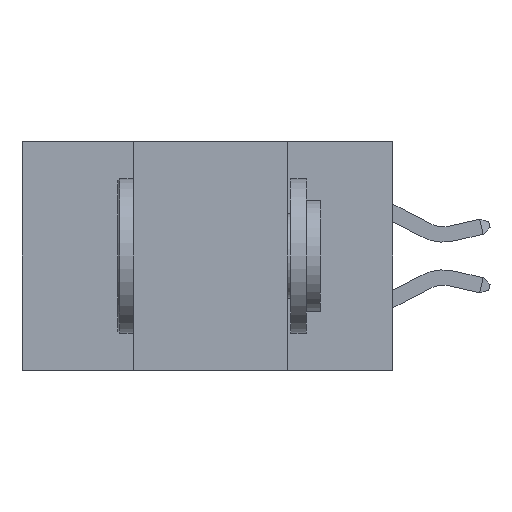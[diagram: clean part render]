
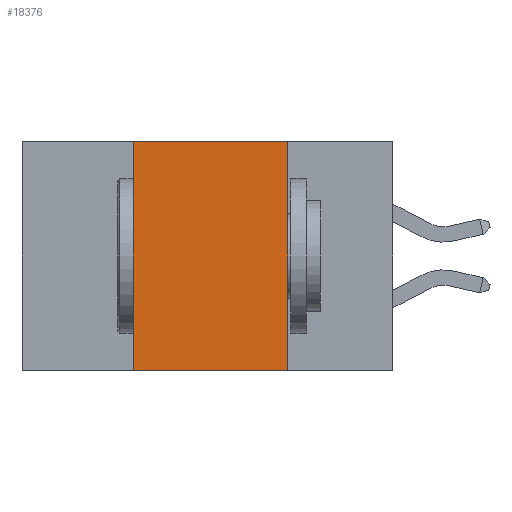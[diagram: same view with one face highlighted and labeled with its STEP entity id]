
A CAD part, left-side view. The second image highlights one B-rep face of the part: STEP entity #18376.
In plain terms, the highlighted planar face has unit normal (-1, 0, 0).
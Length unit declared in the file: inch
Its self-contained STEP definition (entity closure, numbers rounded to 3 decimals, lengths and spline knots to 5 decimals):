
#164 = ORIENTED_EDGE ( 'NONE', *, *, #11476, .F. ) ;
#1396 = EDGE_LOOP ( 'NONE', ( #15743, #164, #21096, #26042 ) ) ;
#4524 = VECTOR ( 'NONE', #17876, 39.37008 ) ;
#4577 = DIRECTION ( 'NONE',  ( 1., 0., 0. ) ) ;
#4940 = LINE ( 'NONE', #6911, #35645 ) ;
#5086 = CARTESIAN_POINT ( 'NONE',  ( 0., 0.6, -0.37 ) ) ;
#5673 = LINE ( 'NONE', #18594, #25231 ) ;
#6781 = DIRECTION ( 'NONE',  ( 0., -1., 0. ) ) ;
#6911 = CARTESIAN_POINT ( 'NONE',  ( 0., 0.6, 0. ) ) ;
#7108 = EDGE_CURVE ( 'NONE', #28613, #36774, #5673, .T. ) ;
#7483 = CARTESIAN_POINT ( 'NONE',  ( 0., 0.6, 0. ) ) ;
#7971 = EDGE_CURVE ( 'NONE', #33020, #36774, #28387, .T. ) ;
#11476 = EDGE_CURVE ( 'NONE', #26983, #28613, #4940, .T. ) ;
#12858 = FACE_OUTER_BOUND ( 'NONE', #1396, .T. ) ;
#13036 = DIRECTION ( 'NONE',  ( 0., 0., -1. ) ) ;
#14779 = CARTESIAN_POINT ( 'NONE',  ( 0., 0.17, -0.37 ) ) ;
#15743 = ORIENTED_EDGE ( 'NONE', *, *, #7108, .F. ) ;
#17222 = VECTOR ( 'NONE', #35237, 39.37008 ) ;
#17876 = DIRECTION ( 'NONE',  ( 0., 0., 1. ) ) ;
#18376 = ADVANCED_FACE ( 'NONE', ( #12858 ), #31241, .F. ) ;
#18594 = CARTESIAN_POINT ( 'NONE',  ( 0., 0.17, 0. ) ) ;
#20415 = CARTESIAN_POINT ( 'NONE',  ( 0., 0.17, 0. ) ) ;
#21096 = ORIENTED_EDGE ( 'NONE', *, *, #25609, .F. ) ;
#23603 = LINE ( 'NONE', #36129, #4524 ) ;
#24091 = CARTESIAN_POINT ( 'NONE',  ( 0., 0.42, 0. ) ) ;
#25231 = VECTOR ( 'NONE', #13036, 39.37008 ) ;
#25609 = EDGE_CURVE ( 'NONE', #33020, #26983, #23603, .T. ) ;
#25943 = AXIS2_PLACEMENT_3D ( 'NONE', #7483, #4577, #37249 ) ;
#26042 = ORIENTED_EDGE ( 'NONE', *, *, #7971, .T. ) ;
#26983 = VERTEX_POINT ( 'NONE', #24091 ) ;
#28387 = LINE ( 'NONE', #5086, #17222 ) ;
#28613 = VERTEX_POINT ( 'NONE', #20415 ) ;
#31204 = CARTESIAN_POINT ( 'NONE',  ( 0., 0.42, -0.37 ) ) ;
#31241 = PLANE ( 'NONE',  #25943 ) ;
#33020 = VERTEX_POINT ( 'NONE', #31204 ) ;
#35237 = DIRECTION ( 'NONE',  ( 0., -1., 0. ) ) ;
#35645 = VECTOR ( 'NONE', #6781, 39.37008 ) ;
#36129 = CARTESIAN_POINT ( 'NONE',  ( 0., 0.42, 0. ) ) ;
#36774 = VERTEX_POINT ( 'NONE', #14779 ) ;
#37249 = DIRECTION ( 'NONE',  ( 0., 0., -1. ) ) ;
